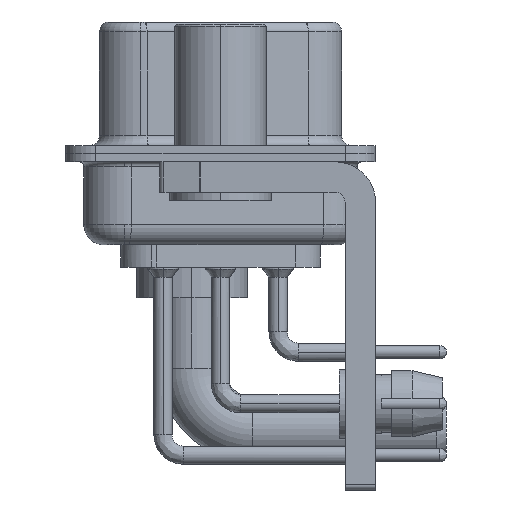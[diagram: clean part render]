
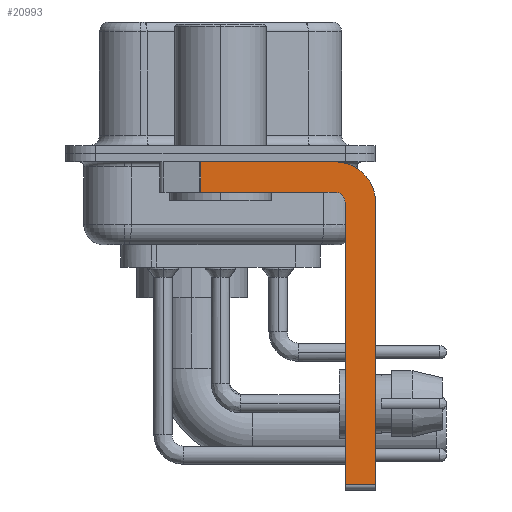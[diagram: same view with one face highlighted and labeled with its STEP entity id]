
A CAD part, left-side view. The second image highlights one B-rep face of the part: STEP entity #20993.
In plain terms, the highlighted planar face has unit normal (-1, 0, 0).
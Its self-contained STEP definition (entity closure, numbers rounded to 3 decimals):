
#131 = EDGE_CURVE ( 'NONE', #3035, #16685, #15334, .T. ) ;
#313 = LINE ( 'NONE', #3356, #3312 ) ;
#389 = CARTESIAN_POINT ( 'NONE',  ( -2.9, 0.978, -0.4 ) ) ;
#814 = DIRECTION ( 'NONE',  ( 1., 0., 0. ) ) ;
#1009 = VECTOR ( 'NONE', #24502, 1000. ) ;
#1299 = VECTOR ( 'NONE', #10577, 1000. ) ;
#2869 = CARTESIAN_POINT ( 'NONE',  ( -2.9, 0.978, -1.9 ) ) ;
#2920 = CARTESIAN_POINT ( 'NONE',  ( -2.9, 0.978, -1.9 ) ) ;
#3035 = VERTEX_POINT ( 'NONE', #37341 ) ;
#3312 = VECTOR ( 'NONE', #15436, 1000. ) ;
#3356 = CARTESIAN_POINT ( 'NONE',  ( -2.9, -7.65, -2.4 ) ) ;
#3546 = AXIS2_PLACEMENT_3D ( 'NONE', #25981, #23905, #27195 ) ;
#4057 = CARTESIAN_POINT ( 'NONE',  ( -2.9, -5.65, -2.4 ) ) ;
#4386 = VERTEX_POINT ( 'NONE', #38652 ) ;
#5863 = EDGE_CURVE ( 'NONE', #16685, #38625, #10459, .T. ) ;
#7138 = ORIENTED_EDGE ( 'NONE', *, *, #16629, .F. ) ;
#7433 = VERTEX_POINT ( 'NONE', #22300 ) ;
#8962 = LINE ( 'NONE', #14899, #1009 ) ;
#9649 = CARTESIAN_POINT ( 'NONE',  ( -2.9, -7.65, -16.35 ) ) ;
#9997 = ORIENTED_EDGE ( 'NONE', *, *, #14668, .F. ) ;
#10256 = CARTESIAN_POINT ( 'NONE',  ( -2.9, -6.15, -16.35 ) ) ;
#10459 = LINE ( 'NONE', #35632, #35487 ) ;
#10577 = DIRECTION ( 'NONE',  ( 0., -1., 0. ) ) ;
#10593 = DIRECTION ( 'NONE',  ( 0., 0., -1. ) ) ;
#12186 = VERTEX_POINT ( 'NONE', #9649 ) ;
#13104 = ORIENTED_EDGE ( 'NONE', *, *, #23245, .T. ) ;
#14668 = EDGE_CURVE ( 'NONE', #29060, #7433, #20187, .T. ) ;
#14854 = VECTOR ( 'NONE', #37216, 1000. ) ;
#14899 = CARTESIAN_POINT ( 'NONE',  ( -2.9, -5.65, -16.35 ) ) ;
#15142 = ORIENTED_EDGE ( 'NONE', *, *, #25820, .F. ) ;
#15334 = CIRCLE ( 'NONE', #15978, 0.5 ) ;
#15436 = DIRECTION ( 'NONE',  ( 0., 0., -1. ) ) ;
#15978 = AXIS2_PLACEMENT_3D ( 'NONE', #35769, #33112, #32711 ) ;
#16233 = CARTESIAN_POINT ( 'NONE',  ( -2.9, -5.65, -1.9 ) ) ;
#16629 = EDGE_CURVE ( 'NONE', #4386, #12186, #313, .T. ) ;
#16685 = VERTEX_POINT ( 'NONE', #16233 ) ;
#17847 = ORIENTED_EDGE ( 'NONE', *, *, #37026, .F. ) ;
#18422 = CARTESIAN_POINT ( 'NONE',  ( -2.9, -6.15, -16.6 ) ) ;
#18637 = LINE ( 'NONE', #18422, #14854 ) ;
#19192 = ORIENTED_EDGE ( 'NONE', *, *, #131, .F. ) ;
#19255 = LINE ( 'NONE', #2920, #32479 ) ;
#20187 = LINE ( 'NONE', #38603, #1299 ) ;
#20993 = ADVANCED_FACE ( 'NONE', ( #26138 ), #28804, .F. ) ;
#22300 = CARTESIAN_POINT ( 'NONE',  ( -2.9, -5.65, -0.4 ) ) ;
#23245 = EDGE_CURVE ( 'NONE', #25535, #12186, #8962, .T. ) ;
#23809 = AXIS2_PLACEMENT_3D ( 'NONE', #4057, #814, #10593 ) ;
#23905 = DIRECTION ( 'NONE',  ( 1., 0., 0. ) ) ;
#24502 = DIRECTION ( 'NONE',  ( 0., -1., 0. ) ) ;
#25535 = VERTEX_POINT ( 'NONE', #10256 ) ;
#25820 = EDGE_CURVE ( 'NONE', #25535, #3035, #18637, .T. ) ;
#25981 = CARTESIAN_POINT ( 'NONE',  ( -2.9, -5.65, -2.4 ) ) ;
#26138 = FACE_OUTER_BOUND ( 'NONE', #39806, .T. ) ;
#27023 = CIRCLE ( 'NONE', #3546, 2. ) ;
#27195 = DIRECTION ( 'NONE',  ( 0., 0., -1. ) ) ;
#27856 = ORIENTED_EDGE ( 'NONE', *, *, #5863, .F. ) ;
#28038 = EDGE_CURVE ( 'NONE', #29060, #38625, #19255, .T. ) ;
#28804 = PLANE ( 'NONE',  #23809 ) ;
#29060 = VERTEX_POINT ( 'NONE', #389 ) ;
#30623 = ORIENTED_EDGE ( 'NONE', *, *, #28038, .T. ) ;
#32479 = VECTOR ( 'NONE', #34792, 1000. ) ;
#32567 = DIRECTION ( 'NONE',  ( 0., 1., 0. ) ) ;
#32711 = DIRECTION ( 'NONE',  ( 0., 0., 1. ) ) ;
#33112 = DIRECTION ( 'NONE',  ( -1., 0., 0. ) ) ;
#34792 = DIRECTION ( 'NONE',  ( 0., 0., -1. ) ) ;
#35487 = VECTOR ( 'NONE', #32567, 1000. ) ;
#35632 = CARTESIAN_POINT ( 'NONE',  ( -2.9, -5.65, -1.9 ) ) ;
#35769 = CARTESIAN_POINT ( 'NONE',  ( -2.9, -5.65, -2.4 ) ) ;
#37026 = EDGE_CURVE ( 'NONE', #7433, #4386, #27023, .T. ) ;
#37216 = DIRECTION ( 'NONE',  ( 0., 0., 1. ) ) ;
#37341 = CARTESIAN_POINT ( 'NONE',  ( -2.9, -6.15, -2.4 ) ) ;
#38603 = CARTESIAN_POINT ( 'NONE',  ( -2.9, 3., -0.4 ) ) ;
#38625 = VERTEX_POINT ( 'NONE', #2869 ) ;
#38652 = CARTESIAN_POINT ( 'NONE',  ( -2.9, -7.65, -2.4 ) ) ;
#39806 = EDGE_LOOP ( 'NONE', ( #9997, #30623, #27856, #19192, #15142, #13104, #7138, #17847 ) ) ;
